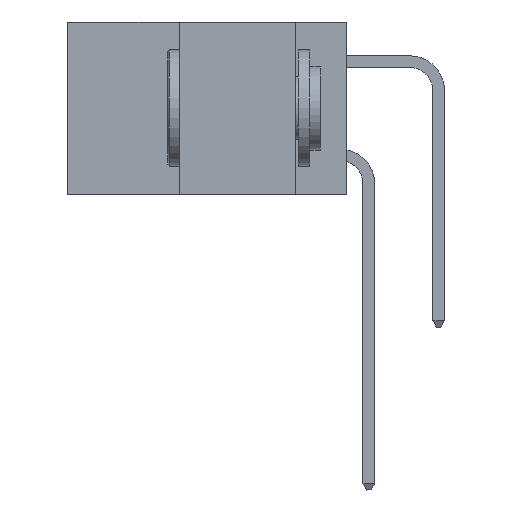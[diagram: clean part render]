
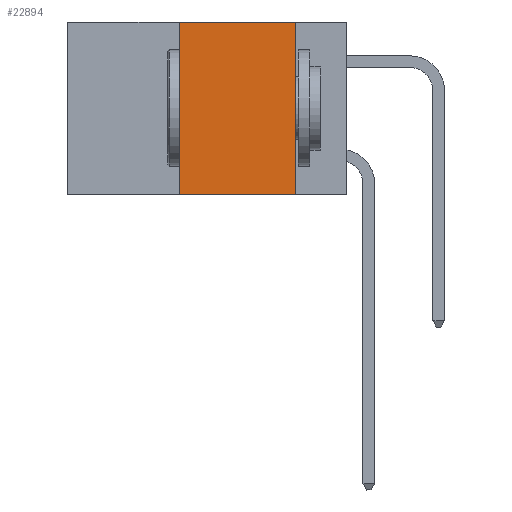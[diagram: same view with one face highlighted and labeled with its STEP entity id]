
A CAD part, left-side view. The second image highlights one B-rep face of the part: STEP entity #22894.
In plain terms, the highlighted planar face has unit normal (-1, 0, 0).
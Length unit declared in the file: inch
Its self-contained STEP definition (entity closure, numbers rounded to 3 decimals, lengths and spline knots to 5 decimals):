
#913 = CARTESIAN_POINT ( 'NONE',  ( 0., 0.11, -0.37 ) ) ;
#944 = VERTEX_POINT ( 'NONE', #20509 ) ;
#2388 = PLANE ( 'NONE',  #25329 ) ;
#3338 = CARTESIAN_POINT ( 'NONE',  ( 0., 0.11, 0. ) ) ;
#4152 = VECTOR ( 'NONE', #12123, 39.37008 ) ;
#4413 = VERTEX_POINT ( 'NONE', #3338 ) ;
#4726 = CARTESIAN_POINT ( 'NONE',  ( 0., 0.36, -0.37 ) ) ;
#5259 = CARTESIAN_POINT ( 'NONE',  ( 0., 0.36, 0. ) ) ;
#6401 = CARTESIAN_POINT ( 'NONE',  ( 0., 0.6, -0.37 ) ) ;
#7133 = DIRECTION ( 'NONE',  ( 1., 0., 0. ) ) ;
#7985 = ORIENTED_EDGE ( 'NONE', *, *, #20410, .F. ) ;
#9440 = ORIENTED_EDGE ( 'NONE', *, *, #23334, .T. ) ;
#12123 = DIRECTION ( 'NONE',  ( 0., 0., 1. ) ) ;
#12453 = CARTESIAN_POINT ( 'NONE',  ( 0., 0.6, 0. ) ) ;
#15031 = LINE ( 'NONE', #6401, #21065 ) ;
#15060 = FACE_OUTER_BOUND ( 'NONE', #17077, .T. ) ;
#15177 = VERTEX_POINT ( 'NONE', #913 ) ;
#17077 = EDGE_LOOP ( 'NONE', ( #19509, #7985, #26847, #9440 ) ) ;
#17925 = DIRECTION ( 'NONE',  ( 0., -1., 0. ) ) ;
#18644 = CARTESIAN_POINT ( 'NONE',  ( 0., 0.6, 0. ) ) ;
#18830 = VERTEX_POINT ( 'NONE', #4726 ) ;
#19323 = CARTESIAN_POINT ( 'NONE',  ( 0., 0.11, 0. ) ) ;
#19509 = ORIENTED_EDGE ( 'NONE', *, *, #23115, .F. ) ;
#20032 = VECTOR ( 'NONE', #26128, 39.37008 ) ;
#20410 = EDGE_CURVE ( 'NONE', #944, #4413, #26793, .T. ) ;
#20509 = CARTESIAN_POINT ( 'NONE',  ( 0., 0.36, 0. ) ) ;
#21065 = VECTOR ( 'NONE', #17925, 39.37008 ) ;
#22294 = VECTOR ( 'NONE', #28232, 39.37008 ) ;
#22894 = ADVANCED_FACE ( 'NONE', ( #15060 ), #2388, .F. ) ;
#23115 = EDGE_CURVE ( 'NONE', #4413, #15177, #25948, .T. ) ;
#23131 = DIRECTION ( 'NONE',  ( 0., 0., -1. ) ) ;
#23334 = EDGE_CURVE ( 'NONE', #18830, #15177, #15031, .T. ) ;
#25329 = AXIS2_PLACEMENT_3D ( 'NONE', #18644, #7133, #23131 ) ;
#25948 = LINE ( 'NONE', #19323, #20032 ) ;
#26128 = DIRECTION ( 'NONE',  ( 0., 0., -1. ) ) ;
#26793 = LINE ( 'NONE', #12453, #22294 ) ;
#26847 = ORIENTED_EDGE ( 'NONE', *, *, #28302, .F. ) ;
#27049 = LINE ( 'NONE', #5259, #4152 ) ;
#28232 = DIRECTION ( 'NONE',  ( 0., -1., 0. ) ) ;
#28302 = EDGE_CURVE ( 'NONE', #18830, #944, #27049, .T. ) ;
